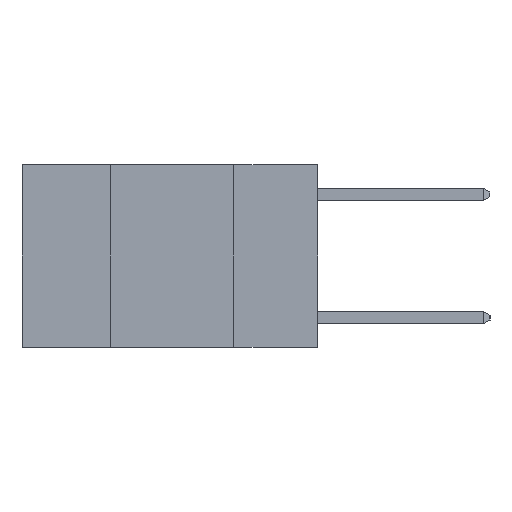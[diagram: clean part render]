
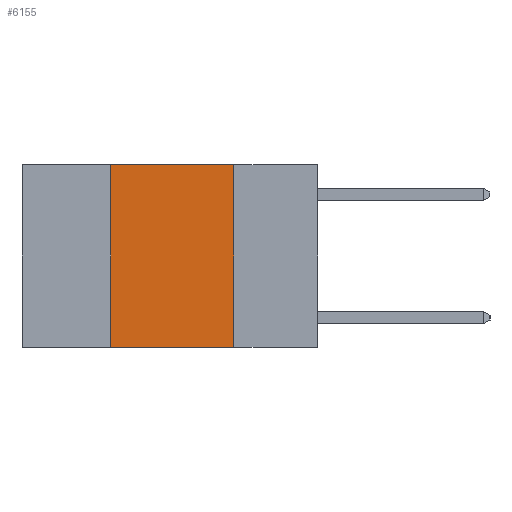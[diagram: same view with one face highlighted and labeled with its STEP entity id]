
A CAD part, left-side view. The second image highlights one B-rep face of the part: STEP entity #6155.
In plain terms, the highlighted planar face has unit normal (-1, 0, 0).
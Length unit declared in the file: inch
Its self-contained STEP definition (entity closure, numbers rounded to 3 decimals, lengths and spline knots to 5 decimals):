
#4 = EDGE_CURVE ( 'NONE', #11674, #2083, #9076, .T. ) ;
#181 = LINE ( 'NONE', #3976, #4815 ) ;
#1018 = DIRECTION ( 'NONE',  ( 0., -1., 0. ) ) ;
#1504 = CARTESIAN_POINT ( 'NONE',  ( 0., 0.17, 0. ) ) ;
#2007 = CARTESIAN_POINT ( 'NONE',  ( 0., 0.6, 0. ) ) ;
#2083 = VERTEX_POINT ( 'NONE', #1504 ) ;
#2275 = CARTESIAN_POINT ( 'NONE',  ( 0., 0.17, -0.37 ) ) ;
#2644 = EDGE_CURVE ( 'NONE', #3674, #11674, #10618, .T. ) ;
#2857 = DIRECTION ( 'NONE',  ( 0., 0., 1. ) ) ;
#2943 = DIRECTION ( 'NONE',  ( 0., 0., -1. ) ) ;
#3094 = VECTOR ( 'NONE', #2857, 39.37008 ) ;
#3129 = CARTESIAN_POINT ( 'NONE',  ( 0., 0.6, 0. ) ) ;
#3577 = ORIENTED_EDGE ( 'NONE', *, *, #8092, .F. ) ;
#3674 = VERTEX_POINT ( 'NONE', #7004 ) ;
#3882 = FACE_OUTER_BOUND ( 'NONE', #9212, .T. ) ;
#3976 = CARTESIAN_POINT ( 'NONE',  ( 0., 0.17, 0. ) ) ;
#4398 = VECTOR ( 'NONE', #1018, 39.37008 ) ;
#4815 = VECTOR ( 'NONE', #4852, 39.37008 ) ;
#4852 = DIRECTION ( 'NONE',  ( 0., 0., -1. ) ) ;
#5313 = VERTEX_POINT ( 'NONE', #2275 ) ;
#5385 = CARTESIAN_POINT ( 'NONE',  ( 0., 0.42, 0. ) ) ;
#5580 = CARTESIAN_POINT ( 'NONE',  ( 0., 0.6, -0.37 ) ) ;
#6155 = ADVANCED_FACE ( 'NONE', ( #3882 ), #6518, .F. ) ;
#6518 = PLANE ( 'NONE',  #10287 ) ;
#6651 = VECTOR ( 'NONE', #9437, 39.37008 ) ;
#6988 = ORIENTED_EDGE ( 'NONE', *, *, #7935, .T. ) ;
#7004 = CARTESIAN_POINT ( 'NONE',  ( 0., 0.42, -0.37 ) ) ;
#7935 = EDGE_CURVE ( 'NONE', #3674, #5313, #11375, .T. ) ;
#8092 = EDGE_CURVE ( 'NONE', #2083, #5313, #181, .T. ) ;
#8270 = ORIENTED_EDGE ( 'NONE', *, *, #4, .F. ) ;
#8346 = DIRECTION ( 'NONE',  ( 1., 0., 0. ) ) ;
#9076 = LINE ( 'NONE', #3129, #6651 ) ;
#9185 = CARTESIAN_POINT ( 'NONE',  ( 0., 0.42, 0. ) ) ;
#9212 = EDGE_LOOP ( 'NONE', ( #3577, #8270, #10979, #6988 ) ) ;
#9437 = DIRECTION ( 'NONE',  ( 0., -1., 0. ) ) ;
#10287 = AXIS2_PLACEMENT_3D ( 'NONE', #2007, #8346, #2943 ) ;
#10618 = LINE ( 'NONE', #9185, #3094 ) ;
#10979 = ORIENTED_EDGE ( 'NONE', *, *, #2644, .F. ) ;
#11375 = LINE ( 'NONE', #5580, #4398 ) ;
#11674 = VERTEX_POINT ( 'NONE', #5385 ) ;
